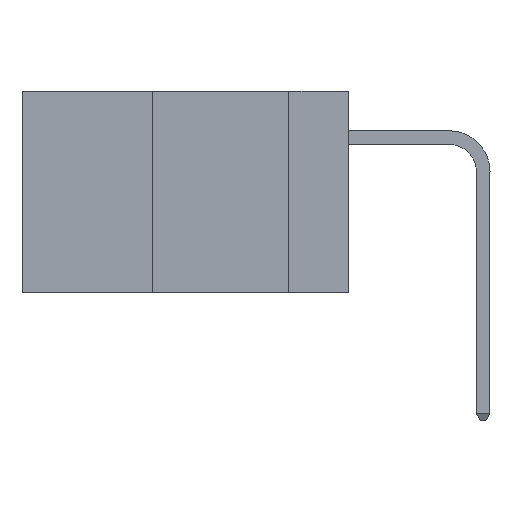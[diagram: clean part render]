
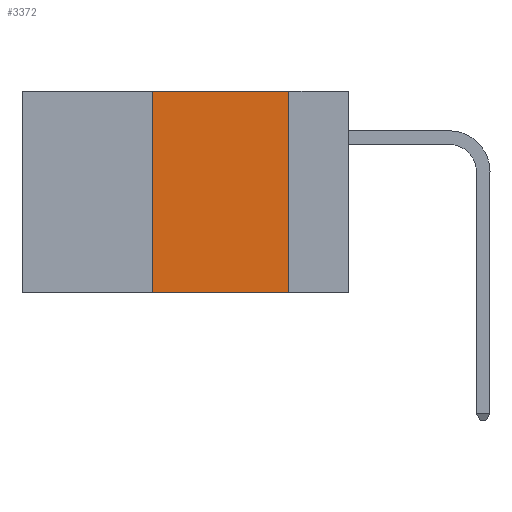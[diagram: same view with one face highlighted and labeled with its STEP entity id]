
A CAD part, left-side view. The second image highlights one B-rep face of the part: STEP entity #3372.
In plain terms, the highlighted planar face has unit normal (-1, 0, 0).
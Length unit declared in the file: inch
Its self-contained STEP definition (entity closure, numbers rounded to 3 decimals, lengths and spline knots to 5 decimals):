
#697 = LINE ( 'NONE', #13167, #1166 ) ;
#1166 = VECTOR ( 'NONE', #32358, 39.37008 ) ;
#2671 = FACE_OUTER_BOUND ( 'NONE', #27620, .T. ) ;
#3372 = ADVANCED_FACE ( 'NONE', ( #2671 ), #13651, .F. ) ;
#3722 = ORIENTED_EDGE ( 'NONE', *, *, #16317, .F. ) ;
#4087 = CARTESIAN_POINT ( 'NONE',  ( 0., 0.6, -0.37 ) ) ;
#4572 = CARTESIAN_POINT ( 'NONE',  ( 0., 0.11, 0. ) ) ;
#6281 = CARTESIAN_POINT ( 'NONE',  ( 0., 0.36, -0.37 ) ) ;
#6413 = DIRECTION ( 'NONE',  ( 0., 0., 1. ) ) ;
#6996 = DIRECTION ( 'NONE',  ( 0., -1., 0. ) ) ;
#7277 = VECTOR ( 'NONE', #6413, 39.37008 ) ;
#7386 = LINE ( 'NONE', #15192, #7277 ) ;
#8595 = ORIENTED_EDGE ( 'NONE', *, *, #28310, .F. ) ;
#8939 = CARTESIAN_POINT ( 'NONE',  ( 0., 0.11, -0.37 ) ) ;
#12271 = ORIENTED_EDGE ( 'NONE', *, *, #32069, .T. ) ;
#12409 = ORIENTED_EDGE ( 'NONE', *, *, #17012, .F. ) ;
#12488 = VECTOR ( 'NONE', #6996, 39.37008 ) ;
#13167 = CARTESIAN_POINT ( 'NONE',  ( 0., 0.6, 0. ) ) ;
#13651 = PLANE ( 'NONE',  #17887 ) ;
#13778 = DIRECTION ( 'NONE',  ( 1., 0., 0. ) ) ;
#15192 = CARTESIAN_POINT ( 'NONE',  ( 0., 0.36, 0. ) ) ;
#15535 = VERTEX_POINT ( 'NONE', #8939 ) ;
#16317 = EDGE_CURVE ( 'NONE', #28671, #26288, #7386, .T. ) ;
#17012 = EDGE_CURVE ( 'NONE', #26288, #22612, #697, .T. ) ;
#17887 = AXIS2_PLACEMENT_3D ( 'NONE', #30234, #13778, #32905 ) ;
#19157 = CARTESIAN_POINT ( 'NONE',  ( 0., 0.11, 0. ) ) ;
#19858 = LINE ( 'NONE', #4087, #12488 ) ;
#20819 = VECTOR ( 'NONE', #21863, 39.37008 ) ;
#21863 = DIRECTION ( 'NONE',  ( 0., 0., -1. ) ) ;
#22612 = VERTEX_POINT ( 'NONE', #4572 ) ;
#26288 = VERTEX_POINT ( 'NONE', #26431 ) ;
#26431 = CARTESIAN_POINT ( 'NONE',  ( 0., 0.36, 0. ) ) ;
#27620 = EDGE_LOOP ( 'NONE', ( #8595, #12409, #3722, #12271 ) ) ;
#28310 = EDGE_CURVE ( 'NONE', #22612, #15535, #36187, .T. ) ;
#28671 = VERTEX_POINT ( 'NONE', #6281 ) ;
#30234 = CARTESIAN_POINT ( 'NONE',  ( 0., 0.6, 0. ) ) ;
#32069 = EDGE_CURVE ( 'NONE', #28671, #15535, #19858, .T. ) ;
#32358 = DIRECTION ( 'NONE',  ( 0., -1., 0. ) ) ;
#32905 = DIRECTION ( 'NONE',  ( 0., 0., -1. ) ) ;
#36187 = LINE ( 'NONE', #19157, #20819 ) ;
